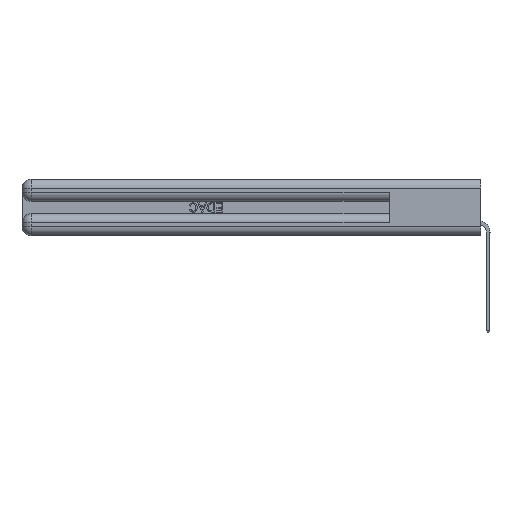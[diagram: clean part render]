
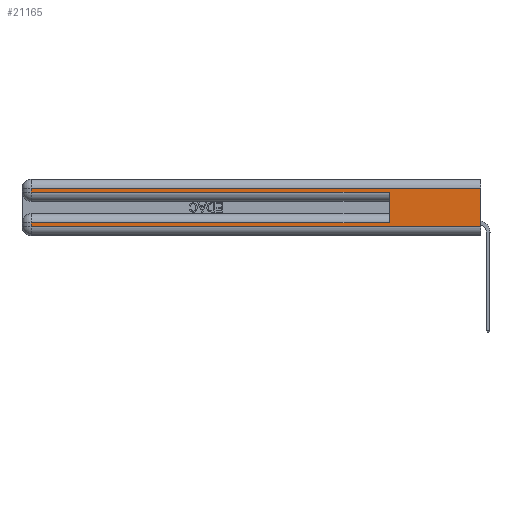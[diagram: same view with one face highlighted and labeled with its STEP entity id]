
A CAD part, left-side view. The second image highlights one B-rep face of the part: STEP entity #21165.
In plain terms, the highlighted planar face has unit normal (-1, 0, 0).
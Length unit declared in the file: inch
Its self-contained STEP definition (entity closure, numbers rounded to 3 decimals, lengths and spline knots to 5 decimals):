
#1900 = CARTESIAN_POINT ( 'NONE',  ( 0., 2.94, 0.31 ) ) ;
#2756 = VECTOR ( 'NONE', #27255, 39.37008 ) ;
#5051 = CARTESIAN_POINT ( 'NONE',  ( 0., 0., 0.37 ) ) ;
#5345 = DIRECTION ( 'NONE',  ( 0., 0., -1. ) ) ;
#6811 = VECTOR ( 'NONE', #43960, 39.37008 ) ;
#7649 = ORIENTED_EDGE ( 'NONE', *, *, #30556, .F. ) ;
#7718 = EDGE_CURVE ( 'NONE', #43114, #11171, #20213, .T. ) ;
#8573 = CARTESIAN_POINT ( 'NONE',  ( 0., 2.94, 0.37 ) ) ;
#9155 = LINE ( 'NONE', #26024, #43705 ) ;
#9697 = LINE ( 'NONE', #34406, #40302 ) ;
#9919 = CARTESIAN_POINT ( 'NONE',  ( 0., 0., 0.31 ) ) ;
#10057 = VERTEX_POINT ( 'NONE', #41527 ) ;
#10094 = DIRECTION ( 'NONE',  ( 0., 0., -1. ) ) ;
#10654 = EDGE_CURVE ( 'NONE', #25235, #24958, #13827, .T. ) ;
#10910 = LINE ( 'NONE', #20400, #19304 ) ;
#10916 = CARTESIAN_POINT ( 'NONE',  ( 0., 2.94, 0.085 ) ) ;
#11171 = VERTEX_POINT ( 'NONE', #13972 ) ;
#11497 = VECTOR ( 'NONE', #33521, 39.37008 ) ;
#11740 = DIRECTION ( 'NONE',  ( 1., 0., 0. ) ) ;
#11790 = EDGE_CURVE ( 'NONE', #25235, #43114, #41552, .T. ) ;
#12907 = ORIENTED_EDGE ( 'NONE', *, *, #42795, .T. ) ;
#13224 = ORIENTED_EDGE ( 'NONE', *, *, #33039, .T. ) ;
#13246 = VECTOR ( 'NONE', #42712, 39.37008 ) ;
#13289 = LINE ( 'NONE', #16628, #2756 ) ;
#13827 = LINE ( 'NONE', #39550, #13246 ) ;
#13972 = CARTESIAN_POINT ( 'NONE',  ( 0., 2.94, 0.06 ) ) ;
#15081 = EDGE_CURVE ( 'NONE', #41815, #20744, #9697, .T. ) ;
#16347 = CARTESIAN_POINT ( 'NONE',  ( 0., 0.6, 0.285 ) ) ;
#16628 = CARTESIAN_POINT ( 'NONE',  ( 0., 0., 0.06 ) ) ;
#16702 = DIRECTION ( 'NONE',  ( 0., 1., 0. ) ) ;
#16961 = ORIENTED_EDGE ( 'NONE', *, *, #15081, .T. ) ;
#18561 = ORIENTED_EDGE ( 'NONE', *, *, #25987, .T. ) ;
#19304 = VECTOR ( 'NONE', #10094, 39.37008 ) ;
#20213 = LINE ( 'NONE', #8573, #6811 ) ;
#20400 = CARTESIAN_POINT ( 'NONE',  ( 0., 2.94, 0.37 ) ) ;
#20686 = DIRECTION ( 'NONE',  ( 0., 1., 0. ) ) ;
#20744 = VERTEX_POINT ( 'NONE', #1900 ) ;
#21053 = LINE ( 'NONE', #5051, #11497 ) ;
#21165 = ADVANCED_FACE ( 'NONE', ( #27351 ), #29340, .F. ) ;
#24910 = VECTOR ( 'NONE', #20686, 39.37008 ) ;
#24958 = VERTEX_POINT ( 'NONE', #16347 ) ;
#25235 = VERTEX_POINT ( 'NONE', #27859 ) ;
#25987 = EDGE_CURVE ( 'NONE', #11171, #10057, #13289, .T. ) ;
#26024 = CARTESIAN_POINT ( 'NONE',  ( 0., 0., 0.285 ) ) ;
#27255 = DIRECTION ( 'NONE',  ( 0., -1., 0. ) ) ;
#27351 = FACE_OUTER_BOUND ( 'NONE', #27949, .T. ) ;
#27859 = CARTESIAN_POINT ( 'NONE',  ( 0., 0.6, 0.085 ) ) ;
#27949 = EDGE_LOOP ( 'NONE', ( #7649, #16961, #13224, #12907, #32591, #29393, #34841, #18561 ) ) ;
#29340 = PLANE ( 'NONE',  #44503 ) ;
#29393 = ORIENTED_EDGE ( 'NONE', *, *, #11790, .T. ) ;
#29437 = VERTEX_POINT ( 'NONE', #39399 ) ;
#29498 = CARTESIAN_POINT ( 'NONE',  ( 0., 0., 0.37 ) ) ;
#30556 = EDGE_CURVE ( 'NONE', #41815, #10057, #21053, .T. ) ;
#32591 = ORIENTED_EDGE ( 'NONE', *, *, #10654, .F. ) ;
#33039 = EDGE_CURVE ( 'NONE', #20744, #29437, #10910, .T. ) ;
#33521 = DIRECTION ( 'NONE',  ( 0., 0., -1. ) ) ;
#34406 = CARTESIAN_POINT ( 'NONE',  ( 0., 0., 0.31 ) ) ;
#34841 = ORIENTED_EDGE ( 'NONE', *, *, #7718, .T. ) ;
#36288 = DIRECTION ( 'NONE',  ( 0., -1., 0. ) ) ;
#37919 = CARTESIAN_POINT ( 'NONE',  ( 0., 0., 0.085 ) ) ;
#39399 = CARTESIAN_POINT ( 'NONE',  ( 0., 2.94, 0.285 ) ) ;
#39550 = CARTESIAN_POINT ( 'NONE',  ( 0., 0.6, 0.145 ) ) ;
#40302 = VECTOR ( 'NONE', #16702, 39.37008 ) ;
#41527 = CARTESIAN_POINT ( 'NONE',  ( 0., 0., 0.06 ) ) ;
#41552 = LINE ( 'NONE', #37919, #24910 ) ;
#41815 = VERTEX_POINT ( 'NONE', #9919 ) ;
#42712 = DIRECTION ( 'NONE',  ( 0., 0., 1. ) ) ;
#42795 = EDGE_CURVE ( 'NONE', #29437, #24958, #9155, .T. ) ;
#43114 = VERTEX_POINT ( 'NONE', #10916 ) ;
#43705 = VECTOR ( 'NONE', #36288, 39.37008 ) ;
#43960 = DIRECTION ( 'NONE',  ( 0., 0., -1. ) ) ;
#44503 = AXIS2_PLACEMENT_3D ( 'NONE', #29498, #11740, #5345 ) ;
